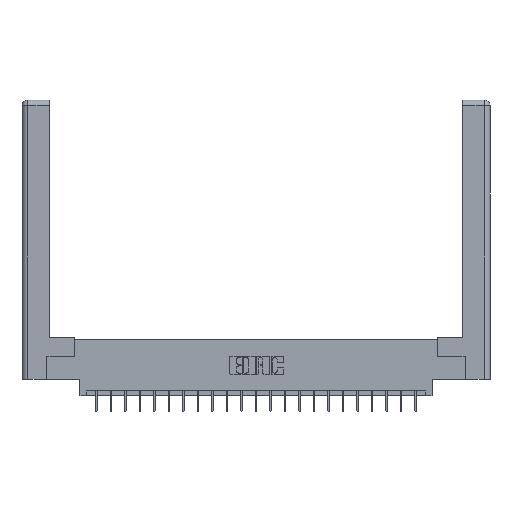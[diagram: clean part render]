
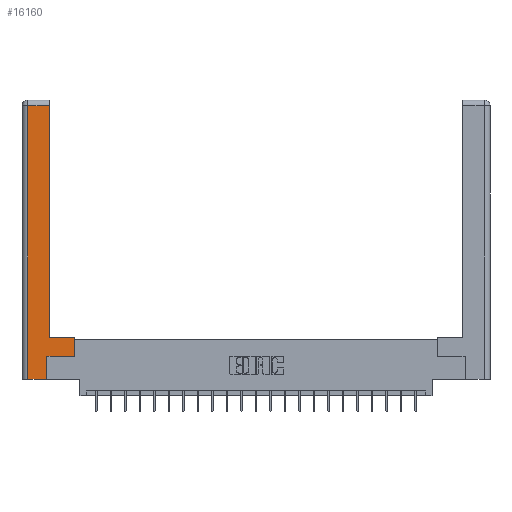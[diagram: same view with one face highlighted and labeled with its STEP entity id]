
A CAD part, top view. The second image highlights one B-rep face of the part: STEP entity #16160.
In plain terms, the highlighted planar face has unit normal (0, 0, 1).
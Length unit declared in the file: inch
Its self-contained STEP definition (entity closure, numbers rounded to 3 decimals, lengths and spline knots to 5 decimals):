
#58 = PLANE ( 'NONE',  #15309 ) ;
#342 = CARTESIAN_POINT ( 'NONE',  ( 0.0615, 2.94, 0. ) ) ;
#502 = VERTEX_POINT ( 'NONE', #12874 ) ;
#833 = FACE_OUTER_BOUND ( 'NONE', #15695, .T. ) ;
#1133 = VERTEX_POINT ( 'NONE', #12621 ) ;
#1579 = CARTESIAN_POINT ( 'NONE',  ( 0.265, 0., 0. ) ) ;
#1669 = CARTESIAN_POINT ( 'NONE',  ( 0.265, 0.245, 0. ) ) ;
#1702 = DIRECTION ( 'NONE',  ( 0., -1., 0. ) ) ;
#2453 = LINE ( 'NONE', #12662, #9489 ) ;
#3351 = DIRECTION ( 'NONE',  ( -1., 0., 0. ) ) ;
#4414 = LINE ( 'NONE', #22219, #4702 ) ;
#4491 = CARTESIAN_POINT ( 'NONE',  ( 0.565, 0.245, 0. ) ) ;
#4626 = EDGE_CURVE ( 'NONE', #6150, #18790, #4414, .T. ) ;
#4702 = VECTOR ( 'NONE', #1702, 39.37008 ) ;
#4755 = VECTOR ( 'NONE', #17121, 39.37008 ) ;
#5669 = CARTESIAN_POINT ( 'NONE',  ( 0.565, 0.45, 0. ) ) ;
#5779 = LINE ( 'NONE', #15028, #12782 ) ;
#6068 = VECTOR ( 'NONE', #9212, 39.37008 ) ;
#6150 = VERTEX_POINT ( 'NONE', #342 ) ;
#6160 = VECTOR ( 'NONE', #21735, 39.37008 ) ;
#6276 = EDGE_CURVE ( 'NONE', #6566, #6150, #20548, .T. ) ;
#6566 = VERTEX_POINT ( 'NONE', #19493 ) ;
#6684 = ORIENTED_EDGE ( 'NONE', *, *, #18832, .T. ) ;
#7655 = CARTESIAN_POINT ( 'NONE',  ( 0.295, 3., 0. ) ) ;
#7806 = LINE ( 'NONE', #7655, #13911 ) ;
#9212 = DIRECTION ( 'NONE',  ( -1., 0., 0. ) ) ;
#9489 = VECTOR ( 'NONE', #19695, 39.37008 ) ;
#9538 = LINE ( 'NONE', #4491, #4755 ) ;
#10617 = LINE ( 'NONE', #5669, #6160 ) ;
#10721 = CARTESIAN_POINT ( 'NONE',  ( 0., 0., 0. ) ) ;
#10821 = VERTEX_POINT ( 'NONE', #15443 ) ;
#11985 = EDGE_CURVE ( 'NONE', #10821, #1133, #2453, .T. ) ;
#12046 = EDGE_CURVE ( 'NONE', #18902, #17298, #14498, .T. ) ;
#12458 = DIRECTION ( 'NONE',  ( 0., 0., -1. ) ) ;
#12621 = CARTESIAN_POINT ( 'NONE',  ( 0.295, 0.45, 0. ) ) ;
#12645 = EDGE_CURVE ( 'NONE', #1133, #6566, #7806, .T. ) ;
#12662 = CARTESIAN_POINT ( 'NONE',  ( 0.295, 0.45, 0. ) ) ;
#12782 = VECTOR ( 'NONE', #18899, 39.37008 ) ;
#12874 = CARTESIAN_POINT ( 'NONE',  ( 0.565, 0.245, 0. ) ) ;
#13009 = CARTESIAN_POINT ( 'NONE',  ( 0.0615, 0., 0. ) ) ;
#13274 = ORIENTED_EDGE ( 'NONE', *, *, #12645, .T. ) ;
#13911 = VECTOR ( 'NONE', #19776, 39.37008 ) ;
#14239 = ORIENTED_EDGE ( 'NONE', *, *, #16896, .T. ) ;
#14498 = LINE ( 'NONE', #16149, #22277 ) ;
#14703 = ORIENTED_EDGE ( 'NONE', *, *, #11985, .T. ) ;
#14981 = ORIENTED_EDGE ( 'NONE', *, *, #12046, .T. ) ;
#15028 = CARTESIAN_POINT ( 'NONE',  ( 0.265, 0., 0. ) ) ;
#15134 = ORIENTED_EDGE ( 'NONE', *, *, #6276, .T. ) ;
#15309 = AXIS2_PLACEMENT_3D ( 'NONE', #10721, #12458, #3351 ) ;
#15443 = CARTESIAN_POINT ( 'NONE',  ( 0.565, 0.45, 0. ) ) ;
#15695 = EDGE_LOOP ( 'NONE', ( #13274, #15134, #20043, #6684, #14981, #21559, #14239, #14703 ) ) ;
#16149 = CARTESIAN_POINT ( 'NONE',  ( 0.265, 0.245, 0. ) ) ;
#16160 = ADVANCED_FACE ( 'NONE', ( #833 ), #58, .F. ) ;
#16896 = EDGE_CURVE ( 'NONE', #502, #10821, #10617, .T. ) ;
#17121 = DIRECTION ( 'NONE',  ( 1., 0., 0. ) ) ;
#17298 = VERTEX_POINT ( 'NONE', #1669 ) ;
#17922 = CARTESIAN_POINT ( 'NONE',  ( 0.0615, 2.94, 0. ) ) ;
#18089 = DIRECTION ( 'NONE',  ( 0., 1., 0. ) ) ;
#18790 = VERTEX_POINT ( 'NONE', #13009 ) ;
#18832 = EDGE_CURVE ( 'NONE', #18790, #18902, #5779, .T. ) ;
#18899 = DIRECTION ( 'NONE',  ( 1., 0., 0. ) ) ;
#18902 = VERTEX_POINT ( 'NONE', #1579 ) ;
#19493 = CARTESIAN_POINT ( 'NONE',  ( 0.295, 2.94, 0. ) ) ;
#19695 = DIRECTION ( 'NONE',  ( -1., 0., 0. ) ) ;
#19776 = DIRECTION ( 'NONE',  ( 0., 1., 0. ) ) ;
#20043 = ORIENTED_EDGE ( 'NONE', *, *, #4626, .T. ) ;
#20548 = LINE ( 'NONE', #17922, #6068 ) ;
#21559 = ORIENTED_EDGE ( 'NONE', *, *, #21785, .T. ) ;
#21735 = DIRECTION ( 'NONE',  ( 0., 1., 0. ) ) ;
#21785 = EDGE_CURVE ( 'NONE', #17298, #502, #9538, .T. ) ;
#22219 = CARTESIAN_POINT ( 'NONE',  ( 0.0615, 0., 0. ) ) ;
#22277 = VECTOR ( 'NONE', #18089, 39.37008 ) ;
